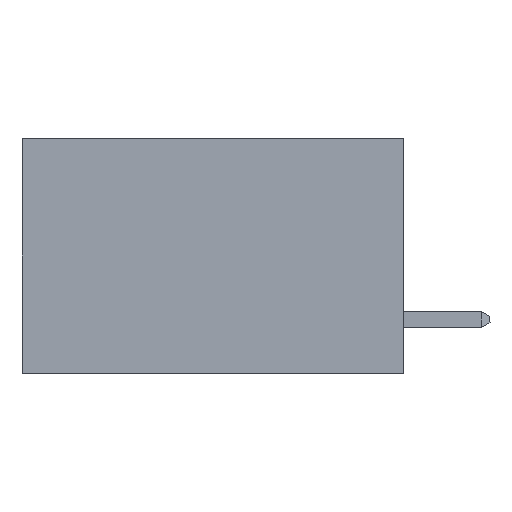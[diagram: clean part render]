
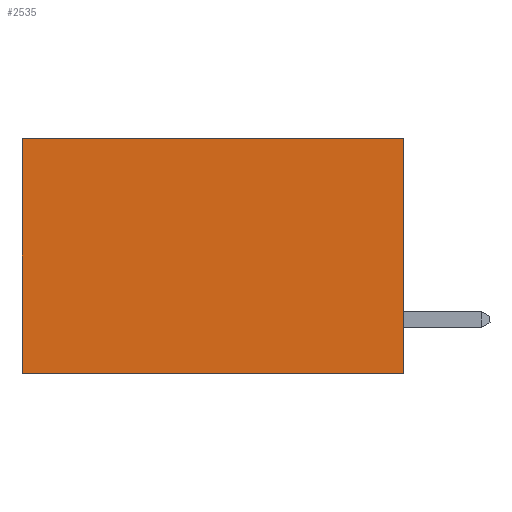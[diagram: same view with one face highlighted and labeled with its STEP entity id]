
A CAD part, left-side view. The second image highlights one B-rep face of the part: STEP entity #2535.
In plain terms, the highlighted planar face has unit normal (-1, 0, 0).
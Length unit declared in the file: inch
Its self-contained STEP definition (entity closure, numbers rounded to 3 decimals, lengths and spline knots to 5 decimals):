
#491 = DIRECTION ( 'NONE',  ( 0., 0., -1. ) ) ;
#1957 = AXIS2_PLACEMENT_3D ( 'NONE', #11959, #22976, #18652 ) ;
#2535 = ADVANCED_FACE ( 'NONE', ( #16570 ), #22953, .F. ) ;
#2748 = LINE ( 'NONE', #6425, #22226 ) ;
#3041 = EDGE_LOOP ( 'NONE', ( #23223, #18623, #10775, #6770 ) ) ;
#3239 = VERTEX_POINT ( 'NONE', #22844 ) ;
#4107 = LINE ( 'NONE', #11619, #17930 ) ;
#4512 = VERTEX_POINT ( 'NONE', #10163 ) ;
#5835 = VECTOR ( 'NONE', #14456, 39.37008 ) ;
#6073 = EDGE_CURVE ( 'NONE', #3239, #16342, #2748, .T. ) ;
#6425 = CARTESIAN_POINT ( 'NONE',  ( 0.2875, 0., 0. ) ) ;
#6665 = VECTOR ( 'NONE', #22733, 39.37008 ) ;
#6770 = ORIENTED_EDGE ( 'NONE', *, *, #16825, .T. ) ;
#8390 = CARTESIAN_POINT ( 'NONE',  ( 0.2875, 0.6, -0.37 ) ) ;
#10163 = CARTESIAN_POINT ( 'NONE',  ( 0.2875, 0.6, 0. ) ) ;
#10775 = ORIENTED_EDGE ( 'NONE', *, *, #6073, .F. ) ;
#11619 = CARTESIAN_POINT ( 'NONE',  ( 0.2875, 0., -0.37 ) ) ;
#11814 = LINE ( 'NONE', #17128, #6665 ) ;
#11959 = CARTESIAN_POINT ( 'NONE',  ( 0.2875, 0., 0. ) ) ;
#12631 = CARTESIAN_POINT ( 'NONE',  ( 0.2875, 0.6, 0. ) ) ;
#14456 = DIRECTION ( 'NONE',  ( 0., 0., -1. ) ) ;
#14669 = VERTEX_POINT ( 'NONE', #8390 ) ;
#14823 = EDGE_CURVE ( 'NONE', #4512, #14669, #20737, .T. ) ;
#15801 = CARTESIAN_POINT ( 'NONE',  ( 0.2875, 0., -0.37 ) ) ;
#16342 = VERTEX_POINT ( 'NONE', #15801 ) ;
#16570 = FACE_OUTER_BOUND ( 'NONE', #3041, .T. ) ;
#16825 = EDGE_CURVE ( 'NONE', #3239, #4512, #11814, .T. ) ;
#17128 = CARTESIAN_POINT ( 'NONE',  ( 0.2875, 0., 0. ) ) ;
#17930 = VECTOR ( 'NONE', #22605, 39.37008 ) ;
#18623 = ORIENTED_EDGE ( 'NONE', *, *, #18808, .F. ) ;
#18652 = DIRECTION ( 'NONE',  ( 0., 0., -1. ) ) ;
#18808 = EDGE_CURVE ( 'NONE', #16342, #14669, #4107, .T. ) ;
#20737 = LINE ( 'NONE', #12631, #5835 ) ;
#22226 = VECTOR ( 'NONE', #491, 39.37008 ) ;
#22605 = DIRECTION ( 'NONE',  ( 0., 1., 0. ) ) ;
#22733 = DIRECTION ( 'NONE',  ( 0., 1., 0. ) ) ;
#22844 = CARTESIAN_POINT ( 'NONE',  ( 0.2875, 0., 0. ) ) ;
#22953 = PLANE ( 'NONE',  #1957 ) ;
#22976 = DIRECTION ( 'NONE',  ( 1., 0., 0. ) ) ;
#23223 = ORIENTED_EDGE ( 'NONE', *, *, #14823, .T. ) ;
